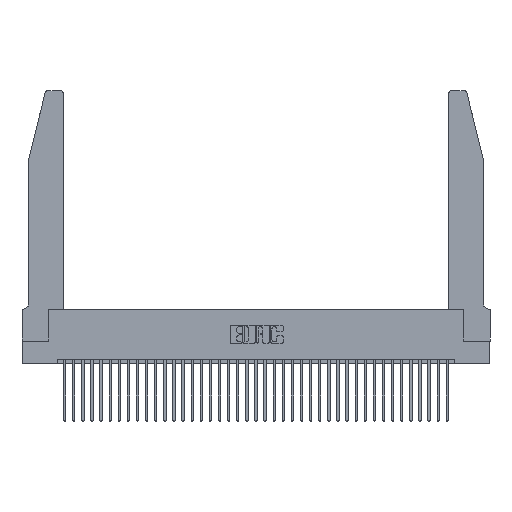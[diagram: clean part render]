
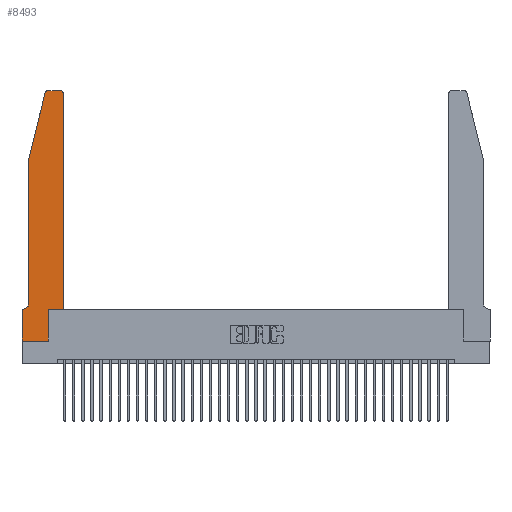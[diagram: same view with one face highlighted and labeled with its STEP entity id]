
A CAD part, top view. The second image highlights one B-rep face of the part: STEP entity #8493.
In plain terms, the highlighted planar face has unit normal (0, 0, 1).
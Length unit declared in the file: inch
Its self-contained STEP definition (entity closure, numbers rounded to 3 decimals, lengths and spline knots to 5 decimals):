
#810 = CARTESIAN_POINT ( 'NONE',  ( 0., 0.35, 0.37 ) ) ;
#971 = EDGE_CURVE ( 'NONE', #17420, #19052, #21397, .T. ) ;
#1081 = AXIS2_PLACEMENT_3D ( 'NONE', #24596, #9788, #24722 ) ;
#1341 = CIRCLE ( 'NONE', #38178, 0.03 ) ;
#1593 = VECTOR ( 'NONE', #33784, 39.37008 ) ;
#1673 = CARTESIAN_POINT ( 'NONE',  ( 0.0755, 0.35, 0.37 ) ) ;
#1857 = ORIENTED_EDGE ( 'NONE', *, *, #24801, .T. ) ;
#1887 = ORIENTED_EDGE ( 'NONE', *, *, #38010, .T. ) ;
#2559 = DIRECTION ( 'NONE',  ( 1., 0., 0. ) ) ;
#2779 = CIRCLE ( 'NONE', #1081, 0.03 ) ;
#2941 = DIRECTION ( 'NONE',  ( 0., 0., 1. ) ) ;
#2993 = VECTOR ( 'NONE', #32899, 39.37008 ) ;
#3286 = CARTESIAN_POINT ( 'NONE',  ( 0.284, 2.75, 0.37 ) ) ;
#3842 = LINE ( 'NONE', #13989, #8977 ) ;
#4256 = CARTESIAN_POINT ( 'NONE',  ( 0., 0.35, 0.37 ) ) ;
#4747 = CARTESIAN_POINT ( 'NONE',  ( 0.0755, 2., 0.37 ) ) ;
#5473 = LINE ( 'NONE', #30342, #21156 ) ;
#5678 = CARTESIAN_POINT ( 'NONE',  ( 0.284, 2.72, 0.37 ) ) ;
#6315 = CARTESIAN_POINT ( 'NONE',  ( 0.2865, 0., 0.37 ) ) ;
#6659 = CARTESIAN_POINT ( 'NONE',  ( 0.4505, 0.35, 0.37 ) ) ;
#7183 = DIRECTION ( 'NONE',  ( 0., 1., 0. ) ) ;
#7578 = EDGE_CURVE ( 'NONE', #28913, #37504, #19002, .T. ) ;
#7709 = AXIS2_PLACEMENT_3D ( 'NONE', #4256, #24658, #33649 ) ;
#8493 = ADVANCED_FACE ( 'NONE', ( #16614 ), #30513, .T. ) ;
#8865 = VECTOR ( 'NONE', #10546, 39.37008 ) ;
#8977 = VECTOR ( 'NONE', #2559, 39.37008 ) ;
#8984 = EDGE_LOOP ( 'NONE', ( #32047, #31087, #20786, #1887, #1857, #21316, #15814, #28111, #34939, #36718, #18624, #14674 ) ) ;
#9788 = DIRECTION ( 'NONE',  ( 0., 0., 1. ) ) ;
#10177 = LINE ( 'NONE', #12107, #29109 ) ;
#10546 = DIRECTION ( 'NONE',  ( -1., 0., 0. ) ) ;
#11041 = AXIS2_PLACEMENT_3D ( 'NONE', #28826, #37635, #13731 ) ;
#11159 = EDGE_CURVE ( 'NONE', #25393, #17676, #37282, .T. ) ;
#11428 = EDGE_CURVE ( 'NONE', #37504, #15626, #26604, .T. ) ;
#12004 = CARTESIAN_POINT ( 'NONE',  ( 0.0755, 2., 0.37 ) ) ;
#12107 = CARTESIAN_POINT ( 'NONE',  ( 0., 0., 0.37 ) ) ;
#13731 = DIRECTION ( 'NONE',  ( -1., 0., 0. ) ) ;
#13989 = CARTESIAN_POINT ( 'NONE',  ( 0.4505, 0.35, 0.37 ) ) ;
#14674 = ORIENTED_EDGE ( 'NONE', *, *, #27683, .T. ) ;
#14712 = DIRECTION ( 'NONE',  ( 1., 0., 0. ) ) ;
#14898 = EDGE_CURVE ( 'NONE', #20504, #30116, #38403, .T. ) ;
#14973 = VECTOR ( 'NONE', #7183, 39.37008 ) ;
#15626 = VERTEX_POINT ( 'NONE', #27022 ) ;
#15814 = ORIENTED_EDGE ( 'NONE', *, *, #11428, .T. ) ;
#16614 = FACE_OUTER_BOUND ( 'NONE', #8984, .T. ) ;
#17420 = VERTEX_POINT ( 'NONE', #6315 ) ;
#17532 = CARTESIAN_POINT ( 'NONE',  ( 0.0755, 2., 0.37 ) ) ;
#17676 = VERTEX_POINT ( 'NONE', #37468 ) ;
#18624 = ORIENTED_EDGE ( 'NONE', *, *, #11159, .T. ) ;
#18865 = DIRECTION ( 'NONE',  ( -1., 0., 0. ) ) ;
#19002 = LINE ( 'NONE', #1673, #8865 ) ;
#19052 = VERTEX_POINT ( 'NONE', #23496 ) ;
#20025 = VECTOR ( 'NONE', #32691, 39.37008 ) ;
#20504 = VERTEX_POINT ( 'NONE', #37066 ) ;
#20786 = ORIENTED_EDGE ( 'NONE', *, *, #14898, .T. ) ;
#21156 = VECTOR ( 'NONE', #18865, 39.37008 ) ;
#21316 = ORIENTED_EDGE ( 'NONE', *, *, #7578, .T. ) ;
#21397 = LINE ( 'NONE', #34137, #14973 ) ;
#21874 = LINE ( 'NONE', #12004, #20025 ) ;
#23496 = CARTESIAN_POINT ( 'NONE',  ( 0.2865, 0.35, 0.37 ) ) ;
#23502 = EDGE_CURVE ( 'NONE', #36470, #38095, #5473, .T. ) ;
#23970 = CARTESIAN_POINT ( 'NONE',  ( 0.0755, 0.42, 0.37 ) ) ;
#24596 = CARTESIAN_POINT ( 'NONE',  ( 0.4205, 2.72, 0.37 ) ) ;
#24658 = DIRECTION ( 'NONE',  ( 0., 0., 1. ) ) ;
#24722 = DIRECTION ( 'NONE',  ( 1., 0., 0. ) ) ;
#24801 = EDGE_CURVE ( 'NONE', #38038, #28913, #36387, .T. ) ;
#24904 = VECTOR ( 'NONE', #32681, 39.37008 ) ;
#25393 = VERTEX_POINT ( 'NONE', #6659 ) ;
#26550 = CARTESIAN_POINT ( 'NONE',  ( 0., 0., 0.37 ) ) ;
#26604 = LINE ( 'NONE', #26550, #2993 ) ;
#27022 = CARTESIAN_POINT ( 'NONE',  ( 0., 0., 0.37 ) ) ;
#27624 = CARTESIAN_POINT ( 'NONE',  ( 0.0055, 0.35, 0.37 ) ) ;
#27683 = EDGE_CURVE ( 'NONE', #17676, #36470, #2779, .T. ) ;
#28111 = ORIENTED_EDGE ( 'NONE', *, *, #30433, .T. ) ;
#28826 = CARTESIAN_POINT ( 'NONE',  ( 0.0055, 0.42, 0.37 ) ) ;
#28913 = VERTEX_POINT ( 'NONE', #27624 ) ;
#29109 = VECTOR ( 'NONE', #14712, 39.37008 ) ;
#29713 = DIRECTION ( 'NONE',  ( 1., 0., 0. ) ) ;
#29745 = EDGE_CURVE ( 'NONE', #38095, #20504, #1341, .T. ) ;
#30116 = VERTEX_POINT ( 'NONE', #4747 ) ;
#30342 = CARTESIAN_POINT ( 'NONE',  ( 0.2605, 2.75, 0.37 ) ) ;
#30433 = EDGE_CURVE ( 'NONE', #15626, #17420, #10177, .T. ) ;
#30513 = PLANE ( 'NONE',  #7709 ) ;
#30640 = CARTESIAN_POINT ( 'NONE',  ( 0.4505, 0.35, 0.37 ) ) ;
#31087 = ORIENTED_EDGE ( 'NONE', *, *, #29745, .T. ) ;
#32047 = ORIENTED_EDGE ( 'NONE', *, *, #23502, .T. ) ;
#32681 = DIRECTION ( 'NONE',  ( -0.239, -0.971, 0. ) ) ;
#32691 = DIRECTION ( 'NONE',  ( 0., -1., 0. ) ) ;
#32899 = DIRECTION ( 'NONE',  ( 0., -1., 0. ) ) ;
#33649 = DIRECTION ( 'NONE',  ( 1., 0., 0. ) ) ;
#33784 = DIRECTION ( 'NONE',  ( 0., 1., 0. ) ) ;
#33937 = EDGE_CURVE ( 'NONE', #19052, #25393, #3842, .T. ) ;
#34137 = CARTESIAN_POINT ( 'NONE',  ( 0.2865, 0.35, 0.37 ) ) ;
#34939 = ORIENTED_EDGE ( 'NONE', *, *, #971, .T. ) ;
#36387 = CIRCLE ( 'NONE', #11041, 0.07 ) ;
#36470 = VERTEX_POINT ( 'NONE', #37836 ) ;
#36718 = ORIENTED_EDGE ( 'NONE', *, *, #33937, .T. ) ;
#37066 = CARTESIAN_POINT ( 'NONE',  ( 0.25487, 2.72718, 0.37 ) ) ;
#37282 = LINE ( 'NONE', #30640, #1593 ) ;
#37468 = CARTESIAN_POINT ( 'NONE',  ( 0.4505, 2.72, 0.37 ) ) ;
#37504 = VERTEX_POINT ( 'NONE', #810 ) ;
#37635 = DIRECTION ( 'NONE',  ( 0., 0., -1. ) ) ;
#37836 = CARTESIAN_POINT ( 'NONE',  ( 0.4205, 2.75, 0.37 ) ) ;
#38010 = EDGE_CURVE ( 'NONE', #30116, #38038, #21874, .T. ) ;
#38038 = VERTEX_POINT ( 'NONE', #23970 ) ;
#38095 = VERTEX_POINT ( 'NONE', #3286 ) ;
#38178 = AXIS2_PLACEMENT_3D ( 'NONE', #5678, #2941, #29713 ) ;
#38403 = LINE ( 'NONE', #17532, #24904 ) ;
